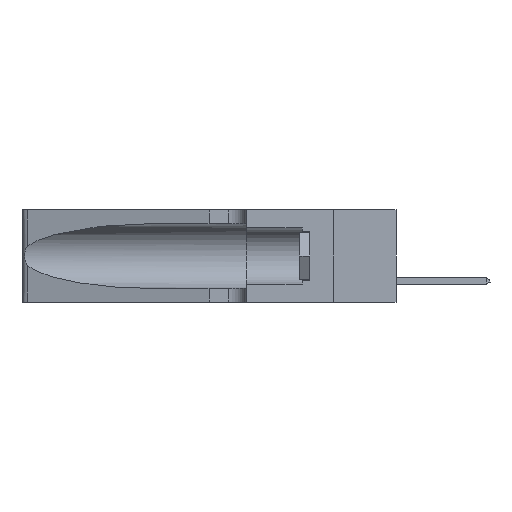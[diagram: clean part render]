
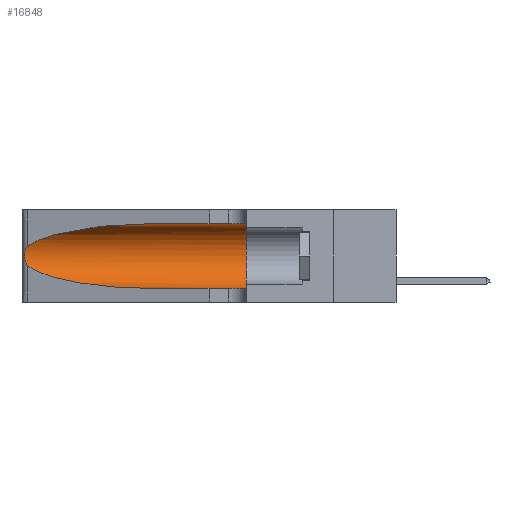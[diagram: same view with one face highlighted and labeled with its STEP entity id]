
A CAD part, left-side view. The second image highlights one B-rep face of the part: STEP entity #16848.
In plain terms, the highlighted cylindrical face has radius 3.308 mm (diameter 6.617 mm), a partial arc.
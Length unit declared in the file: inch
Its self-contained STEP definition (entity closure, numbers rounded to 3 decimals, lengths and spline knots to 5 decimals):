
#92 = DIRECTION ( 'NONE',  ( 0., -1., 0. ) ) ;
#832 = CIRCLE ( 'NONE', #9178, 0.13025 ) ;
#944 = EDGE_CURVE ( 'NONE', #12922, #17652, #9397, .T. ) ;
#1276 = AXIS2_PLACEMENT_3D ( 'NONE', #22502, #92, #15604 ) ;
#2171 = CARTESIAN_POINT ( 'NONE',  ( 0.2373, 1.15595, 0.28018 ) ) ;
#3131 = ORIENTED_EDGE ( 'NONE', *, *, #24046, .T. ) ;
#3506 =( BOUNDED_CURVE ( )  B_SPLINE_CURVE ( 3, ( #17683, #15448, #2171, #28725 ),
 .UNSPECIFIED., .F., .T. ) 
 B_SPLINE_CURVE_WITH_KNOTS ( ( 4, 4 ),
 ( 1.5708, 2.84003 ),
 .UNSPECIFIED. ) 
 CURVE ( )  GEOMETRIC_REPRESENTATION_ITEM ( )  RATIONAL_B_SPLINE_CURVE ( ( 1., 0.87, 0.87, 1. ) ) 
 REPRESENTATION_ITEM ( '' )  );
#3636 = CARTESIAN_POINT ( 'NONE',  ( 0.25487, 1.22718, 0.22369 ) ) ;
#4815 = VERTEX_POINT ( 'NONE', #7649 ) ;
#6207 = CARTESIAN_POINT ( 'NONE',  ( 0.26075, 1.23896, 0.19203 ) ) ;
#6297 = CARTESIAN_POINT ( 'NONE',  ( 0.25487, 1.22718, 0.22369 ) ) ;
#6754 = CARTESIAN_POINT ( 'NONE',  ( 0.18966, 0.96281, 0.05475 ) ) ;
#7146 = ORIENTED_EDGE ( 'NONE', *, *, #26523, .T. ) ;
#7649 = CARTESIAN_POINT ( 'NONE',  ( 0.25487, 1.22718, 0.14631 ) ) ;
#7854 = DIRECTION ( 'NONE',  ( 0., 1., 0. ) ) ;
#7927 = DIRECTION ( 'NONE',  ( 0., -1., 0. ) ) ;
#8417 = CARTESIAN_POINT ( 'NONE',  ( 0.1305, 0.35, 0.31525 ) ) ;
#8473 = CARTESIAN_POINT ( 'NONE',  ( 0.25555, 1.22993, 0.14849 ) ) ;
#8707 = VERTEX_POINT ( 'NONE', #3636 ) ;
#9178 = AXIS2_PLACEMENT_3D ( 'NONE', #25624, #7854, #10035 ) ;
#9397 = LINE ( 'NONE', #16838, #24047 ) ;
#10035 = DIRECTION ( 'NONE',  ( 0., 0., 1. ) ) ;
#10540 = CARTESIAN_POINT ( 'NONE',  ( 0.25555, 1.22994, 0.2215 ) ) ;
#10817 = CARTESIAN_POINT ( 'NONE',  ( 0.26018, 1.23835, 0.19895 ) ) ;
#11002 = CARTESIAN_POINT ( 'NONE',  ( 0.2373, 1.15595, 0.08982 ) ) ;
#11283 = CARTESIAN_POINT ( 'NONE',  ( 0.1305, 0.72297, 0.05475 ) ) ;
#11455 = VERTEX_POINT ( 'NONE', #23243 ) ;
#12102 = CARTESIAN_POINT ( 'NONE',  ( 0.1305, 0.35, 0.05475 ) ) ;
#12253 = VECTOR ( 'NONE', #13095, 39.37008 ) ;
#12922 = VERTEX_POINT ( 'NONE', #25244 ) ;
#13044 = CARTESIAN_POINT ( 'NONE',  ( 0.25789, 1.23486, 0.15765 ) ) ;
#13095 = DIRECTION ( 'NONE',  ( 0., -1., 0. ) ) ;
#13675 = ORIENTED_EDGE ( 'NONE', *, *, #944, .T. ) ;
#15224 = CARTESIAN_POINT ( 'NONE',  ( 0.25639, 1.23184, 0.21858 ) ) ;
#15313 = CARTESIAN_POINT ( 'NONE',  ( 0.25487, 1.22718, 0.14631 ) ) ;
#15448 = CARTESIAN_POINT ( 'NONE',  ( 0.18966, 0.96281, 0.31525 ) ) ;
#15604 = DIRECTION ( 'NONE',  ( 0., 0., -1. ) ) ;
#16705 = EDGE_CURVE ( 'NONE', #8707, #4815, #24235, .T. ) ;
#16816 = CYLINDRICAL_SURFACE ( 'NONE', #1276, 0.13025 ) ;
#16838 = CARTESIAN_POINT ( 'NONE',  ( 0.1305, 1.61858, 0.05475 ) ) ;
#16848 = ADVANCED_FACE ( 'NONE', ( #22040 ), #16816, .F. ) ;
#17363 = CARTESIAN_POINT ( 'NONE',  ( 0.25787, 1.23484, 0.2124 ) ) ;
#17652 = VERTEX_POINT ( 'NONE', #12102 ) ;
#17683 = CARTESIAN_POINT ( 'NONE',  ( 0.1305, 0.72297, 0.31525 ) ) ;
#18189 = ORIENTED_EDGE ( 'NONE', *, *, #20658, .F. ) ;
#19612 = CARTESIAN_POINT ( 'NONE',  ( 0.25854, 1.2359, 0.20912 ) ) ;
#20621 = LINE ( 'NONE', #24008, #12253 ) ;
#20658 = EDGE_CURVE ( 'NONE', #11455, #23899, #20621, .T. ) ;
#21852 = CARTESIAN_POINT ( 'NONE',  ( 0.26017, 1.23833, 0.17102 ) ) ;
#22040 = FACE_OUTER_BOUND ( 'NONE', #25806, .T. ) ;
#22502 = CARTESIAN_POINT ( 'NONE',  ( 0.1305, 1.61858, 0.185 ) ) ;
#23243 = CARTESIAN_POINT ( 'NONE',  ( 0.1305, 0.72297, 0.31525 ) ) ;
#23899 = VERTEX_POINT ( 'NONE', #8417 ) ;
#24008 = CARTESIAN_POINT ( 'NONE',  ( 0.1305, 1.61858, 0.31525 ) ) ;
#24046 = EDGE_CURVE ( 'NONE', #11455, #8707, #3506, .T. ) ;
#24047 = VECTOR ( 'NONE', #7927, 39.37008 ) ;
#24050 = CARTESIAN_POINT ( 'NONE',  ( 0.26075, 1.23896, 0.178 ) ) ;
#24235 = B_SPLINE_CURVE_WITH_KNOTS ( 'NONE', 3,
 ( #6297, #10540, #15224, #17363, #19612, #10817, #6207, #24050, #21852, #26123, #13044, #24242, #8473, #15313 ),
 .UNSPECIFIED., .F., .F.,
 ( 4, 2, 2, 2, 2, 2, 4 ),
 ( 0., 0.00027, 0.00053, 0.00107, 0.0016, 0.00187, 0.00214 ),
 .UNSPECIFIED. ) ;
#24242 = CARTESIAN_POINT ( 'NONE',  ( 0.25639, 1.23186, 0.15144 ) ) ;
#24601 = ORIENTED_EDGE ( 'NONE', *, *, #16705, .T. ) ;
#25035 = EDGE_CURVE ( 'NONE', #23899, #17652, #832, .T. ) ;
#25244 = CARTESIAN_POINT ( 'NONE',  ( 0.1305, 0.72297, 0.05475 ) ) ;
#25624 = CARTESIAN_POINT ( 'NONE',  ( 0.1305, 0.35, 0.185 ) ) ;
#25806 = EDGE_LOOP ( 'NONE', ( #3131, #24601, #7146, #13675, #27918, #18189 ) ) ;
#26123 = CARTESIAN_POINT ( 'NONE',  ( 0.25856, 1.23593, 0.16098 ) ) ;
#26485 = CARTESIAN_POINT ( 'NONE',  ( 0.25487, 1.22718, 0.14631 ) ) ;
#26523 = EDGE_CURVE ( 'NONE', #4815, #12922, #27265, .T. ) ;
#27265 =( BOUNDED_CURVE ( )  B_SPLINE_CURVE ( 3, ( #26485, #11002, #6754, #11283 ),
 .UNSPECIFIED., .F., .T. ) 
 B_SPLINE_CURVE_WITH_KNOTS ( ( 4, 4 ),
 ( 3.44316, 4.71239 ),
 .UNSPECIFIED. ) 
 CURVE ( )  GEOMETRIC_REPRESENTATION_ITEM ( )  RATIONAL_B_SPLINE_CURVE ( ( 1., 0.87, 0.87, 1. ) ) 
 REPRESENTATION_ITEM ( '' )  );
#27918 = ORIENTED_EDGE ( 'NONE', *, *, #25035, .F. ) ;
#28725 = CARTESIAN_POINT ( 'NONE',  ( 0.25487, 1.22718, 0.22369 ) ) ;
